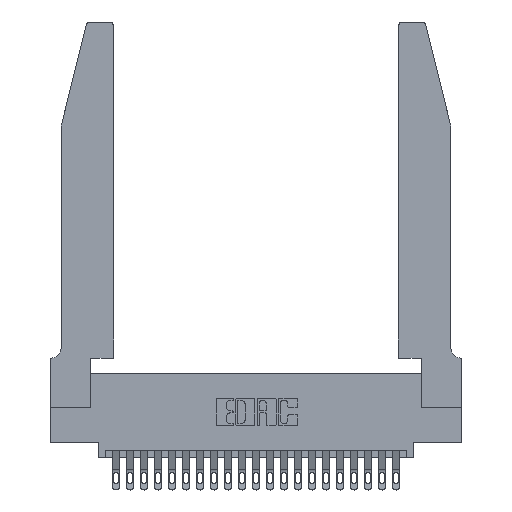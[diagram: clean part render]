
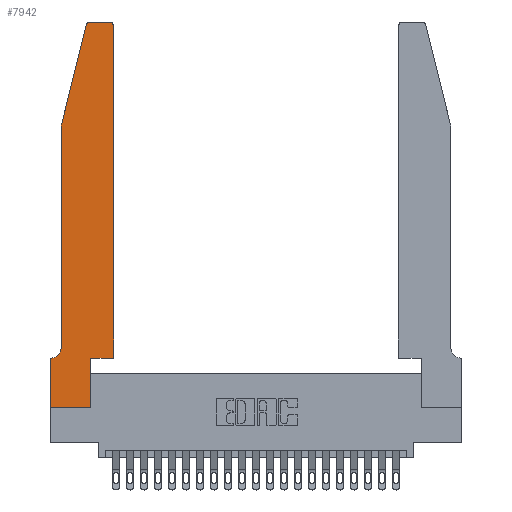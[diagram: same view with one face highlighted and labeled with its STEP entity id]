
A CAD part, top view. The second image highlights one B-rep face of the part: STEP entity #7942.
In plain terms, the highlighted planar face has unit normal (0, 0, 1).
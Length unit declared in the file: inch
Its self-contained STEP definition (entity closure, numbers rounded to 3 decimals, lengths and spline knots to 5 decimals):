
#28 = ORIENTED_EDGE ( 'NONE', *, *, #23657, .T. ) ;
#111 = CARTESIAN_POINT ( 'NONE',  ( 0.4205, 2.72, 0.37 ) ) ;
#446 = VECTOR ( 'NONE', #4835, 39.37008 ) ;
#650 = DIRECTION ( 'NONE',  ( -1., 0., 0. ) ) ;
#703 = CARTESIAN_POINT ( 'NONE',  ( 0.0055, 0.42, 0.37 ) ) ;
#908 = CARTESIAN_POINT ( 'NONE',  ( 0.2865, 0., 0.37 ) ) ;
#1162 = DIRECTION ( 'NONE',  ( 1., 0., 0. ) ) ;
#1354 = CARTESIAN_POINT ( 'NONE',  ( 0.2605, 2.75, 0.37 ) ) ;
#1400 = ORIENTED_EDGE ( 'NONE', *, *, #23580, .T. ) ;
#1537 = LINE ( 'NONE', #17843, #16264 ) ;
#2115 = DIRECTION ( 'NONE',  ( 1., 0., 0. ) ) ;
#2132 = AXIS2_PLACEMENT_3D ( 'NONE', #2483, #4553, #17761 ) ;
#2144 = CARTESIAN_POINT ( 'NONE',  ( 0.0755, 2., 0.37 ) ) ;
#2214 = CARTESIAN_POINT ( 'NONE',  ( 0.2865, 0.35, 0.37 ) ) ;
#2483 = CARTESIAN_POINT ( 'NONE',  ( 0., 0.35, 0.37 ) ) ;
#2716 = DIRECTION ( 'NONE',  ( -1., 0., 0. ) ) ;
#3053 = CARTESIAN_POINT ( 'NONE',  ( 0.0755, 2., 0.37 ) ) ;
#3206 = CARTESIAN_POINT ( 'NONE',  ( 0., 0., 0.37 ) ) ;
#3265 = VERTEX_POINT ( 'NONE', #11756 ) ;
#3408 = ORIENTED_EDGE ( 'NONE', *, *, #11169, .T. ) ;
#3811 = ORIENTED_EDGE ( 'NONE', *, *, #8626, .T. ) ;
#3845 = ORIENTED_EDGE ( 'NONE', *, *, #24043, .T. ) ;
#3987 = LINE ( 'NONE', #9105, #17903 ) ;
#4195 = ORIENTED_EDGE ( 'NONE', *, *, #6019, .T. ) ;
#4450 = DIRECTION ( 'NONE',  ( 0., 0., 1. ) ) ;
#4491 = CARTESIAN_POINT ( 'NONE',  ( 0.0055, 0.35, 0.37 ) ) ;
#4532 = VECTOR ( 'NONE', #22942, 39.37008 ) ;
#4553 = DIRECTION ( 'NONE',  ( 0., 0., 1. ) ) ;
#4563 = VECTOR ( 'NONE', #16418, 39.37008 ) ;
#4835 = DIRECTION ( 'NONE',  ( 0., 1., 0. ) ) ;
#4927 = VERTEX_POINT ( 'NONE', #23617 ) ;
#5151 = DIRECTION ( 'NONE',  ( 1., 0., 0. ) ) ;
#5176 = CARTESIAN_POINT ( 'NONE',  ( 0.284, 2.75, 0.37 ) ) ;
#5249 = ORIENTED_EDGE ( 'NONE', *, *, #10842, .T. ) ;
#5448 = ORIENTED_EDGE ( 'NONE', *, *, #16561, .T. ) ;
#5819 = LINE ( 'NONE', #18024, #446 ) ;
#6019 = EDGE_CURVE ( 'NONE', #13554, #22479, #7904, .T. ) ;
#6062 = ORIENTED_EDGE ( 'NONE', *, *, #18387, .T. ) ;
#6148 = ORIENTED_EDGE ( 'NONE', *, *, #21912, .T. ) ;
#6306 = EDGE_LOOP ( 'NONE', ( #6062, #4195, #3845, #28, #3811, #5448, #7038, #7286, #1400, #5249, #6148, #3408 ) ) ;
#6653 = CARTESIAN_POINT ( 'NONE',  ( 0.0755, 0.42, 0.37 ) ) ;
#7038 = ORIENTED_EDGE ( 'NONE', *, *, #19460, .T. ) ;
#7286 = ORIENTED_EDGE ( 'NONE', *, *, #19428, .T. ) ;
#7293 = LINE ( 'NONE', #1354, #11755 ) ;
#7459 = VECTOR ( 'NONE', #23826, 39.37008 ) ;
#7551 = LINE ( 'NONE', #12913, #16875 ) ;
#7904 = CIRCLE ( 'NONE', #21453, 0.03 ) ;
#7942 = ADVANCED_FACE ( 'NONE', ( #17711 ), #15921, .T. ) ;
#8148 = VECTOR ( 'NONE', #1162, 39.37008 ) ;
#8626 = EDGE_CURVE ( 'NONE', #14039, #13351, #19427, .T. ) ;
#9099 = CARTESIAN_POINT ( 'NONE',  ( 0., 0.35, 0.37 ) ) ;
#9105 = CARTESIAN_POINT ( 'NONE',  ( 0.4505, 0.35, 0.37 ) ) ;
#9169 = LINE ( 'NONE', #3053, #4563 ) ;
#9368 = VERTEX_POINT ( 'NONE', #23514 ) ;
#10842 = EDGE_CURVE ( 'NONE', #19181, #3265, #3987, .T. ) ;
#11020 = CARTESIAN_POINT ( 'NONE',  ( 0.4505, 0.35, 0.37 ) ) ;
#11169 = EDGE_CURVE ( 'NONE', #9368, #4927, #20738, .T. ) ;
#11755 = VECTOR ( 'NONE', #18558, 39.37008 ) ;
#11756 = CARTESIAN_POINT ( 'NONE',  ( 0.4505, 0.35, 0.37 ) ) ;
#12667 = VERTEX_POINT ( 'NONE', #3206 ) ;
#12913 = CARTESIAN_POINT ( 'NONE',  ( 0., 0., 0.37 ) ) ;
#13351 = VERTEX_POINT ( 'NONE', #4491 ) ;
#13388 = AXIS2_PLACEMENT_3D ( 'NONE', #111, #13729, #2115 ) ;
#13554 = VERTEX_POINT ( 'NONE', #5176 ) ;
#13729 = DIRECTION ( 'NONE',  ( 0., 0., 1. ) ) ;
#14039 = VERTEX_POINT ( 'NONE', #6653 ) ;
#14268 = DIRECTION ( 'NONE',  ( 0., 0., -1. ) ) ;
#14607 = CARTESIAN_POINT ( 'NONE',  ( 0.25487, 2.72718, 0.37 ) ) ;
#14769 = DIRECTION ( 'NONE',  ( 0., -1., 0. ) ) ;
#15835 = CARTESIAN_POINT ( 'NONE',  ( 0.284, 2.72, 0.37 ) ) ;
#15921 = PLANE ( 'NONE',  #2132 ) ;
#16264 = VECTOR ( 'NONE', #650, 39.37008 ) ;
#16418 = DIRECTION ( 'NONE',  ( 0., -1., 0. ) ) ;
#16561 = EDGE_CURVE ( 'NONE', #13351, #16686, #1537, .T. ) ;
#16686 = VERTEX_POINT ( 'NONE', #9099 ) ;
#16875 = VECTOR ( 'NONE', #14769, 39.37008 ) ;
#17672 = DIRECTION ( 'NONE',  ( 1., 0., 0. ) ) ;
#17711 = FACE_OUTER_BOUND ( 'NONE', #6306, .T. ) ;
#17761 = DIRECTION ( 'NONE',  ( 1., 0., 0. ) ) ;
#17843 = CARTESIAN_POINT ( 'NONE',  ( 0.0755, 0.35, 0.37 ) ) ;
#17903 = VECTOR ( 'NONE', #5151, 39.37008 ) ;
#18024 = CARTESIAN_POINT ( 'NONE',  ( 0.2865, 0.35, 0.37 ) ) ;
#18387 = EDGE_CURVE ( 'NONE', #4927, #13554, #7293, .T. ) ;
#18558 = DIRECTION ( 'NONE',  ( -1., 0., 0. ) ) ;
#19181 = VERTEX_POINT ( 'NONE', #2214 ) ;
#19427 = CIRCLE ( 'NONE', #24407, 0.07 ) ;
#19428 = EDGE_CURVE ( 'NONE', #12667, #21253, #22873, .T. ) ;
#19460 = EDGE_CURVE ( 'NONE', #16686, #12667, #7551, .T. ) ;
#20098 = LINE ( 'NONE', #2144, #4532 ) ;
#20477 = CARTESIAN_POINT ( 'NONE',  ( 0.0755, 2., 0.37 ) ) ;
#20738 = CIRCLE ( 'NONE', #13388, 0.03 ) ;
#20775 = VERTEX_POINT ( 'NONE', #20477 ) ;
#21253 = VERTEX_POINT ( 'NONE', #908 ) ;
#21453 = AXIS2_PLACEMENT_3D ( 'NONE', #15835, #4450, #17672 ) ;
#21912 = EDGE_CURVE ( 'NONE', #3265, #9368, #22211, .T. ) ;
#22211 = LINE ( 'NONE', #11020, #7459 ) ;
#22479 = VERTEX_POINT ( 'NONE', #14607 ) ;
#22873 = LINE ( 'NONE', #23794, #8148 ) ;
#22942 = DIRECTION ( 'NONE',  ( -0.239, -0.971, 0. ) ) ;
#23514 = CARTESIAN_POINT ( 'NONE',  ( 0.4505, 2.72, 0.37 ) ) ;
#23580 = EDGE_CURVE ( 'NONE', #21253, #19181, #5819, .T. ) ;
#23617 = CARTESIAN_POINT ( 'NONE',  ( 0.4205, 2.75, 0.37 ) ) ;
#23657 = EDGE_CURVE ( 'NONE', #20775, #14039, #9169, .T. ) ;
#23794 = CARTESIAN_POINT ( 'NONE',  ( 0., 0., 0.37 ) ) ;
#23826 = DIRECTION ( 'NONE',  ( 0., 1., 0. ) ) ;
#24043 = EDGE_CURVE ( 'NONE', #22479, #20775, #20098, .T. ) ;
#24407 = AXIS2_PLACEMENT_3D ( 'NONE', #703, #14268, #2716 ) ;
